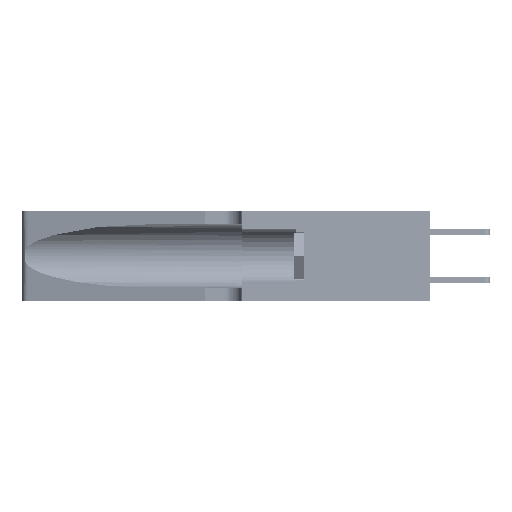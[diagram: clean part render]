
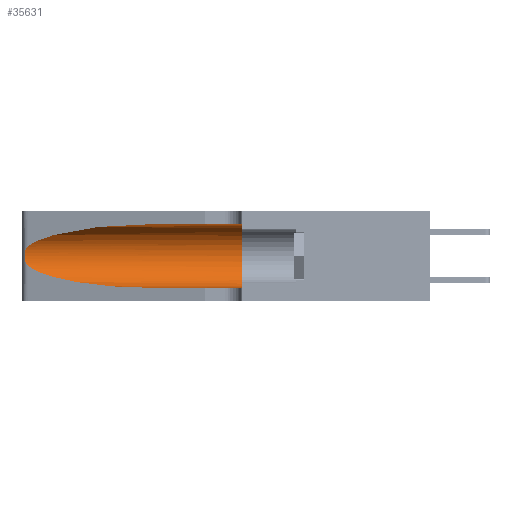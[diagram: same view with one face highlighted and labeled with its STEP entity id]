
A CAD part, left-side view. The second image highlights one B-rep face of the part: STEP entity #35631.
In plain terms, the highlighted cylindrical face has radius 3.308 mm (diameter 6.617 mm), a partial arc.
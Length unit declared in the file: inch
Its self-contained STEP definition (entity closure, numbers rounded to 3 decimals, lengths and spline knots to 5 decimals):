
#300 = DIRECTION ( 'NONE',  ( 0., -1., 0. ) ) ;
#660 = EDGE_CURVE ( 'NONE', #39590, #11480, #24837, .T. ) ;
#1865 = VERTEX_POINT ( 'NONE', #2437 ) ;
#2437 = CARTESIAN_POINT ( 'NONE',  ( 0.25487, 1.22718, 0.14631 ) ) ;
#2926 = ORIENTED_EDGE ( 'NONE', *, *, #660, .F. ) ;
#3134 = DIRECTION ( 'NONE',  ( 0., -1., 0. ) ) ;
#4549 = CARTESIAN_POINT ( 'NONE',  ( 0.25856, 1.23593, 0.16098 ) ) ;
#5357 = LINE ( 'NONE', #26953, #39363 ) ;
#5488 = ORIENTED_EDGE ( 'NONE', *, *, #34220, .T. ) ;
#5690 = EDGE_LOOP ( 'NONE', ( #5488, #13116, #20260, #37022, #2926, #12650 ) ) ;
#5919 = DIRECTION ( 'NONE',  ( 0., 1., 0. ) ) ;
#7042 = VERTEX_POINT ( 'NONE', #9749 ) ;
#8016 = CARTESIAN_POINT ( 'NONE',  ( 0.26075, 1.23896, 0.178 ) ) ;
#8652 = CARTESIAN_POINT ( 'NONE',  ( 0.2373, 1.15595, 0.08982 ) ) ;
#9749 = CARTESIAN_POINT ( 'NONE',  ( 0.1305, 0.72297, 0.31525 ) ) ;
#9867 = CARTESIAN_POINT ( 'NONE',  ( 0.1305, 0.35, 0.185 ) ) ;
#11480 = VERTEX_POINT ( 'NONE', #46891 ) ;
#11523 = CARTESIAN_POINT ( 'NONE',  ( 0.25789, 1.23486, 0.15765 ) ) ;
#12650 = ORIENTED_EDGE ( 'NONE', *, *, #34041, .F. ) ;
#12777 = CARTESIAN_POINT ( 'NONE',  ( 0.1305, 0.72297, 0.05475 ) ) ;
#13116 = ORIENTED_EDGE ( 'NONE', *, *, #29020, .T. ) ;
#13611 =( BOUNDED_CURVE ( )  B_SPLINE_CURVE ( 3, ( #19569, #8652, #34212, #12777 ),
 .UNSPECIFIED., .F., .F. ) 
 B_SPLINE_CURVE_WITH_KNOTS ( ( 4, 4 ),
 ( 3.44316, 4.71239 ),
 .UNSPECIFIED. ) 
 CURVE ( )  GEOMETRIC_REPRESENTATION_ITEM ( )  RATIONAL_B_SPLINE_CURVE ( ( 1., 0.87, 0.87, 1. ) ) 
 REPRESENTATION_ITEM ( '' )  );
#14903 = CARTESIAN_POINT ( 'NONE',  ( 0.25487, 1.22718, 0.22369 ) ) ;
#15041 = DIRECTION ( 'NONE',  ( 0., 0., -1. ) ) ;
#16600 = CARTESIAN_POINT ( 'NONE',  ( 0.1305, 0.35, 0.31525 ) ) ;
#17860 = CARTESIAN_POINT ( 'NONE',  ( 0.2373, 1.15595, 0.28018 ) ) ;
#18641 = CARTESIAN_POINT ( 'NONE',  ( 0.25854, 1.2359, 0.20912 ) ) ;
#18804 = CARTESIAN_POINT ( 'NONE',  ( 0.25487, 1.22718, 0.22369 ) ) ;
#19218 = EDGE_CURVE ( 'NONE', #1865, #41665, #13611, .T. ) ;
#19569 = CARTESIAN_POINT ( 'NONE',  ( 0.25487, 1.22718, 0.14631 ) ) ;
#20260 = ORIENTED_EDGE ( 'NONE', *, *, #19218, .T. ) ;
#22289 = CARTESIAN_POINT ( 'NONE',  ( 0.25639, 1.23186, 0.15144 ) ) ;
#22342 = CYLINDRICAL_SURFACE ( 'NONE', #28257, 0.13025 ) ;
#22440 = CARTESIAN_POINT ( 'NONE',  ( 0.26075, 1.23896, 0.19203 ) ) ;
#23045 = VECTOR ( 'NONE', #3134, 39.37008 ) ;
#24837 = CIRCLE ( 'NONE', #38200, 0.13025 ) ;
#24850 = CARTESIAN_POINT ( 'NONE',  ( 0.1305, 1.61858, 0.31525 ) ) ;
#26493 = VERTEX_POINT ( 'NONE', #14903 ) ;
#26953 = CARTESIAN_POINT ( 'NONE',  ( 0.1305, 1.61858, 0.05475 ) ) ;
#26968 =( BOUNDED_CURVE ( )  B_SPLINE_CURVE ( 3, ( #43644, #39863, #17860, #39549 ),
 .UNSPECIFIED., .F., .T. ) 
 B_SPLINE_CURVE_WITH_KNOTS ( ( 4, 4 ),
 ( 1.5708, 2.84003 ),
 .UNSPECIFIED. ) 
 CURVE ( )  GEOMETRIC_REPRESENTATION_ITEM ( )  RATIONAL_B_SPLINE_CURVE ( ( 1., 0.87, 0.87, 1. ) ) 
 REPRESENTATION_ITEM ( '' )  );
#28257 = AXIS2_PLACEMENT_3D ( 'NONE', #36277, #300, #15041 ) ;
#28302 = CARTESIAN_POINT ( 'NONE',  ( 0.1305, 0.72297, 0.05475 ) ) ;
#29020 = EDGE_CURVE ( 'NONE', #26493, #1865, #43787, .T. ) ;
#29589 = CARTESIAN_POINT ( 'NONE',  ( 0.25639, 1.23184, 0.21858 ) ) ;
#30051 = CARTESIAN_POINT ( 'NONE',  ( 0.26018, 1.23835, 0.19895 ) ) ;
#32444 = EDGE_CURVE ( 'NONE', #41665, #11480, #5357, .T. ) ;
#33690 = FACE_OUTER_BOUND ( 'NONE', #5690, .T. ) ;
#34041 = EDGE_CURVE ( 'NONE', #7042, #39590, #41198, .T. ) ;
#34212 = CARTESIAN_POINT ( 'NONE',  ( 0.18966, 0.96281, 0.05475 ) ) ;
#34220 = EDGE_CURVE ( 'NONE', #7042, #26493, #26968, .T. ) ;
#35240 = DIRECTION ( 'NONE',  ( 0., 0., 1. ) ) ;
#35631 = ADVANCED_FACE ( 'NONE', ( #33690 ), #22342, .F. ) ;
#36277 = CARTESIAN_POINT ( 'NONE',  ( 0.1305, 1.61858, 0.185 ) ) ;
#36695 = CARTESIAN_POINT ( 'NONE',  ( 0.26017, 1.23833, 0.17102 ) ) ;
#36860 = CARTESIAN_POINT ( 'NONE',  ( 0.25787, 1.23484, 0.2124 ) ) ;
#37022 = ORIENTED_EDGE ( 'NONE', *, *, #32444, .T. ) ;
#38200 = AXIS2_PLACEMENT_3D ( 'NONE', #9867, #5919, #35240 ) ;
#39363 = VECTOR ( 'NONE', #41205, 39.37008 ) ;
#39549 = CARTESIAN_POINT ( 'NONE',  ( 0.25487, 1.22718, 0.22369 ) ) ;
#39590 = VERTEX_POINT ( 'NONE', #16600 ) ;
#39863 = CARTESIAN_POINT ( 'NONE',  ( 0.18966, 0.96281, 0.31525 ) ) ;
#40198 = CARTESIAN_POINT ( 'NONE',  ( 0.25555, 1.22993, 0.14849 ) ) ;
#41198 = LINE ( 'NONE', #24850, #23045 ) ;
#41205 = DIRECTION ( 'NONE',  ( 0., -1., 0. ) ) ;
#41665 = VERTEX_POINT ( 'NONE', #28302 ) ;
#43644 = CARTESIAN_POINT ( 'NONE',  ( 0.1305, 0.72297, 0.31525 ) ) ;
#43787 = B_SPLINE_CURVE_WITH_KNOTS ( 'NONE', 3,
 ( #18804, #44114, #29589, #36860, #18641, #30051, #22440, #8016, #36695, #4549, #11523, #22289, #40198, #44278 ),
 .UNSPECIFIED., .F., .F.,
 ( 4, 2, 2, 2, 2, 2, 4 ),
 ( 0., 0.00027, 0.00053, 0.00107, 0.0016, 0.00187, 0.00214 ),
 .UNSPECIFIED. ) ;
#44114 = CARTESIAN_POINT ( 'NONE',  ( 0.25555, 1.22994, 0.2215 ) ) ;
#44278 = CARTESIAN_POINT ( 'NONE',  ( 0.25487, 1.22718, 0.14631 ) ) ;
#46891 = CARTESIAN_POINT ( 'NONE',  ( 0.1305, 0.35, 0.05475 ) ) ;
